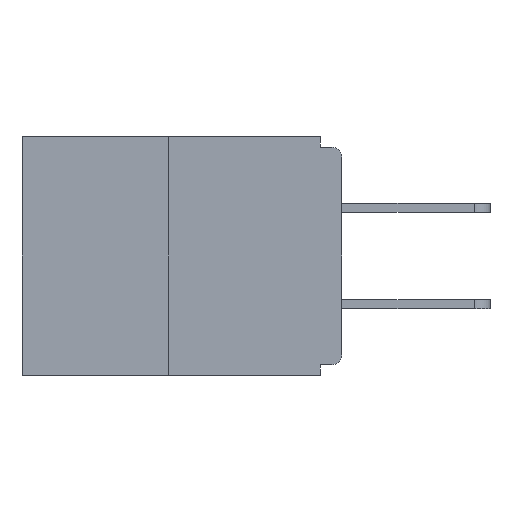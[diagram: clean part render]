
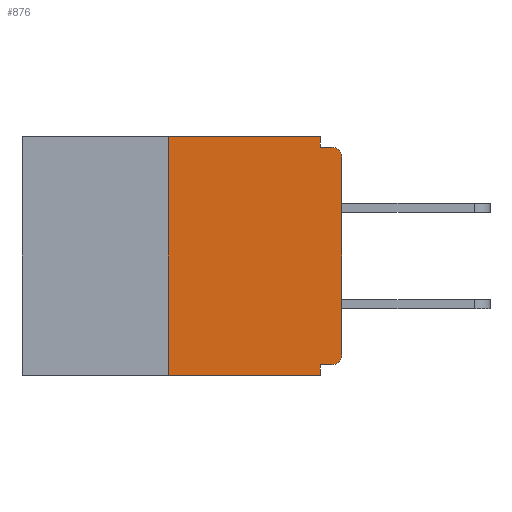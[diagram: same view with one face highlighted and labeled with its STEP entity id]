
A CAD part, left-side view. The second image highlights one B-rep face of the part: STEP entity #876.
In plain terms, the highlighted planar face has unit normal (-1, 0, 0).
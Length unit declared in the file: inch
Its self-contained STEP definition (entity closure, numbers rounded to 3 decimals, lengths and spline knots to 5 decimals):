
#166 = CARTESIAN_POINT ( 'NONE',  ( 0., 0., -0.328 ) ) ;
#245 = EDGE_CURVE ( 'NONE', #10743, #13282, #618, .T. ) ;
#618 = CIRCLE ( 'NONE', #5006, 0.015 ) ;
#710 = ORIENTED_EDGE ( 'NONE', *, *, #8274, .T. ) ;
#741 = ORIENTED_EDGE ( 'NONE', *, *, #9110, .T. ) ;
#869 = CARTESIAN_POINT ( 'NONE',  ( 0., 0.46, 0. ) ) ;
#876 = ADVANCED_FACE ( 'NONE', ( #1929 ), #7711, .F. ) ;
#1059 = VERTEX_POINT ( 'NONE', #10777 ) ;
#1214 = EDGE_CURVE ( 'NONE', #1059, #5745, #9100, .T. ) ;
#1346 = CARTESIAN_POINT ( 'NONE',  ( 0., 0.25, 0. ) ) ;
#1349 = CARTESIAN_POINT ( 'NONE',  ( 0., 0.031, -0.343 ) ) ;
#1566 = ORIENTED_EDGE ( 'NONE', *, *, #5053, .F. ) ;
#1793 = CIRCLE ( 'NONE', #13541, 0.015 ) ;
#1909 = VECTOR ( 'NONE', #6805, 39.37008 ) ;
#1929 = FACE_OUTER_BOUND ( 'NONE', #2365, .T. ) ;
#2193 = EDGE_CURVE ( 'NONE', #5745, #13441, #6589, .T. ) ;
#2245 = LINE ( 'NONE', #13217, #1909 ) ;
#2285 = LINE ( 'NONE', #8826, #5636 ) ;
#2344 = DIRECTION ( 'NONE',  ( 0., 0., -1. ) ) ;
#2365 = EDGE_LOOP ( 'NONE', ( #5701, #7069, #710, #5201, #7576, #741, #7588, #10045, #10550, #1566 ) ) ;
#2806 = CARTESIAN_POINT ( 'NONE',  ( 0., 0.25, 0. ) ) ;
#2922 = VECTOR ( 'NONE', #7651, 39.37008 ) ;
#3297 = CARTESIAN_POINT ( 'NONE',  ( 0., 0.015, -0.03 ) ) ;
#3748 = CARTESIAN_POINT ( 'NONE',  ( 0., 0.031, -0.343 ) ) ;
#3887 = EDGE_CURVE ( 'NONE', #5140, #13282, #2285, .T. ) ;
#3899 = VERTEX_POINT ( 'NONE', #10081 ) ;
#4502 = DIRECTION ( 'NONE',  ( 0., 0., 1. ) ) ;
#4676 = DIRECTION ( 'NONE',  ( 1., 0., 0. ) ) ;
#4714 = EDGE_CURVE ( 'NONE', #12714, #10395, #5121, .T. ) ;
#4757 = DIRECTION ( 'NONE',  ( 0., -1., 0. ) ) ;
#4834 = VECTOR ( 'NONE', #4757, 39.37008 ) ;
#5006 = AXIS2_PLACEMENT_3D ( 'NONE', #3297, #7598, #2344 ) ;
#5053 = EDGE_CURVE ( 'NONE', #10395, #5140, #2245, .T. ) ;
#5121 = LINE ( 'NONE', #869, #6108 ) ;
#5140 = VERTEX_POINT ( 'NONE', #11292 ) ;
#5201 = ORIENTED_EDGE ( 'NONE', *, *, #2193, .F. ) ;
#5265 = LINE ( 'NONE', #1346, #5943 ) ;
#5636 = VECTOR ( 'NONE', #10035, 39.37008 ) ;
#5701 = ORIENTED_EDGE ( 'NONE', *, *, #4714, .F. ) ;
#5745 = VERTEX_POINT ( 'NONE', #10130 ) ;
#5943 = VECTOR ( 'NONE', #8769, 39.37008 ) ;
#6108 = VECTOR ( 'NONE', #6246, 39.37008 ) ;
#6246 = DIRECTION ( 'NONE',  ( 0., -1., 0. ) ) ;
#6416 = CARTESIAN_POINT ( 'NONE',  ( 0., 0.015, -0.015 ) ) ;
#6589 = LINE ( 'NONE', #3748, #9558 ) ;
#6805 = DIRECTION ( 'NONE',  ( 0., 0., -1. ) ) ;
#6834 = CARTESIAN_POINT ( 'NONE',  ( 0., 0., 0. ) ) ;
#6888 = VERTEX_POINT ( 'NONE', #13715 ) ;
#7067 = DIRECTION ( 'NONE',  ( 0., 0., -1. ) ) ;
#7069 = ORIENTED_EDGE ( 'NONE', *, *, #12988, .F. ) ;
#7394 = DIRECTION ( 'NONE',  ( 0., 0., -1. ) ) ;
#7576 = ORIENTED_EDGE ( 'NONE', *, *, #1214, .F. ) ;
#7588 = ORIENTED_EDGE ( 'NONE', *, *, #12665, .T. ) ;
#7598 = DIRECTION ( 'NONE',  ( -1., 0., 0. ) ) ;
#7651 = DIRECTION ( 'NONE',  ( 0., 1., 0. ) ) ;
#7711 = PLANE ( 'NONE',  #12904 ) ;
#7845 = LINE ( 'NONE', #9134, #4834 ) ;
#8274 = EDGE_CURVE ( 'NONE', #6888, #13441, #7845, .T. ) ;
#8546 = CARTESIAN_POINT ( 'NONE',  ( 0., 0.015, -0.313 ) ) ;
#8769 = DIRECTION ( 'NONE',  ( 0., 0., 1. ) ) ;
#8826 = CARTESIAN_POINT ( 'NONE',  ( 0., 0., -0.015 ) ) ;
#8890 = CARTESIAN_POINT ( 'NONE',  ( 0., 0.031, 0. ) ) ;
#9100 = LINE ( 'NONE', #166, #2922 ) ;
#9110 = EDGE_CURVE ( 'NONE', #1059, #3899, #1793, .T. ) ;
#9134 = CARTESIAN_POINT ( 'NONE',  ( 0., 0.46, -0.343 ) ) ;
#9215 = CARTESIAN_POINT ( 'NONE',  ( 0., 0., -0.03 ) ) ;
#9558 = VECTOR ( 'NONE', #7067, 39.37008 ) ;
#9996 = DIRECTION ( 'NONE',  ( 0., 0., -1. ) ) ;
#10035 = DIRECTION ( 'NONE',  ( 0., -1., 0. ) ) ;
#10045 = ORIENTED_EDGE ( 'NONE', *, *, #245, .T. ) ;
#10081 = CARTESIAN_POINT ( 'NONE',  ( 0., 0., -0.313 ) ) ;
#10130 = CARTESIAN_POINT ( 'NONE',  ( 0., 0.031, -0.328 ) ) ;
#10395 = VERTEX_POINT ( 'NONE', #8890 ) ;
#10550 = ORIENTED_EDGE ( 'NONE', *, *, #3887, .F. ) ;
#10743 = VERTEX_POINT ( 'NONE', #9215 ) ;
#10777 = CARTESIAN_POINT ( 'NONE',  ( 0., 0.015, -0.328 ) ) ;
#11292 = CARTESIAN_POINT ( 'NONE',  ( 0., 0.031, -0.015 ) ) ;
#11647 = LINE ( 'NONE', #6834, #12829 ) ;
#12039 = CARTESIAN_POINT ( 'NONE',  ( 0., 0.46, 0. ) ) ;
#12665 = EDGE_CURVE ( 'NONE', #3899, #10743, #11647, .T. ) ;
#12714 = VERTEX_POINT ( 'NONE', #2806 ) ;
#12829 = VECTOR ( 'NONE', #4502, 39.37008 ) ;
#12882 = DIRECTION ( 'NONE',  ( -1., 0., 0. ) ) ;
#12904 = AXIS2_PLACEMENT_3D ( 'NONE', #12039, #4676, #9996 ) ;
#12988 = EDGE_CURVE ( 'NONE', #6888, #12714, #5265, .T. ) ;
#13217 = CARTESIAN_POINT ( 'NONE',  ( 0., 0.031, 0. ) ) ;
#13282 = VERTEX_POINT ( 'NONE', #6416 ) ;
#13441 = VERTEX_POINT ( 'NONE', #1349 ) ;
#13541 = AXIS2_PLACEMENT_3D ( 'NONE', #8546, #12882, #7394 ) ;
#13715 = CARTESIAN_POINT ( 'NONE',  ( 0., 0.25, -0.343 ) ) ;
